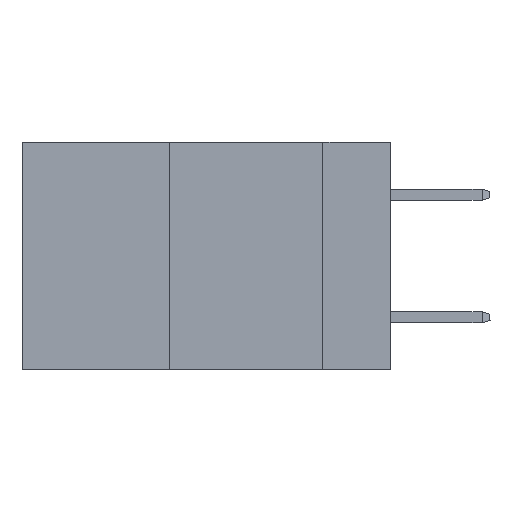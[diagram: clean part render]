
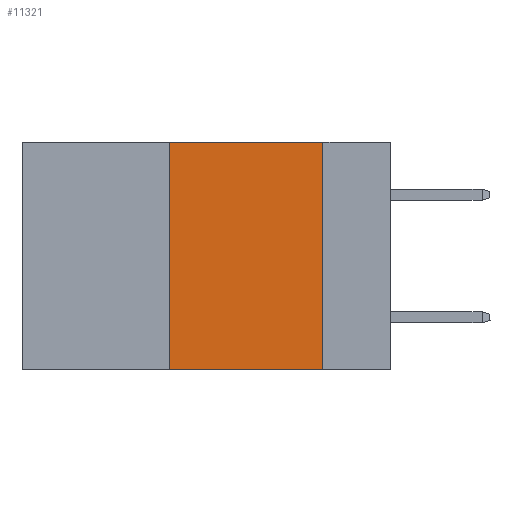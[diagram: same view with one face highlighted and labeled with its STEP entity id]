
A CAD part, left-side view. The second image highlights one B-rep face of the part: STEP entity #11321.
In plain terms, the highlighted planar face has unit normal (-1, 0, 0).
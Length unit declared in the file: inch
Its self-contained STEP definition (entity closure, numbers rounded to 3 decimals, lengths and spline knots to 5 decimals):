
#44 = LINE ( 'NONE', #5130, #1860 ) ;
#545 = CARTESIAN_POINT ( 'NONE',  ( 0., 0.6, 0. ) ) ;
#884 = EDGE_CURVE ( 'NONE', #6959, #10726, #12597, .T. ) ;
#888 = EDGE_CURVE ( 'NONE', #15827, #6959, #13977, .T. ) ;
#1541 = FACE_OUTER_BOUND ( 'NONE', #12123, .T. ) ;
#1860 = VECTOR ( 'NONE', #12966, 39.37008 ) ;
#2761 = ORIENTED_EDGE ( 'NONE', *, *, #884, .F. ) ;
#2857 = AXIS2_PLACEMENT_3D ( 'NONE', #14589, #6434, #11677 ) ;
#2940 = LINE ( 'NONE', #3061, #4414 ) ;
#3061 = CARTESIAN_POINT ( 'NONE',  ( 0., 0.6, -0.37 ) ) ;
#4271 = EDGE_CURVE ( 'NONE', #15827, #9612, #2940, .T. ) ;
#4414 = VECTOR ( 'NONE', #5964, 39.37008 ) ;
#5130 = CARTESIAN_POINT ( 'NONE',  ( 0., 0.11, 0. ) ) ;
#5546 = EDGE_CURVE ( 'NONE', #10726, #9612, #44, .T. ) ;
#5548 = ORIENTED_EDGE ( 'NONE', *, *, #888, .F. ) ;
#5964 = DIRECTION ( 'NONE',  ( 0., -1., 0. ) ) ;
#6434 = DIRECTION ( 'NONE',  ( 1., 0., 0. ) ) ;
#6959 = VERTEX_POINT ( 'NONE', #12556 ) ;
#7631 = VECTOR ( 'NONE', #11240, 39.37008 ) ;
#8489 = ORIENTED_EDGE ( 'NONE', *, *, #4271, .T. ) ;
#9612 = VERTEX_POINT ( 'NONE', #15588 ) ;
#10726 = VERTEX_POINT ( 'NONE', #15538 ) ;
#11240 = DIRECTION ( 'NONE',  ( 0., -1., 0. ) ) ;
#11321 = ADVANCED_FACE ( 'NONE', ( #1541 ), #14647, .F. ) ;
#11677 = DIRECTION ( 'NONE',  ( 0., 0., -1. ) ) ;
#12123 = EDGE_LOOP ( 'NONE', ( #16167, #2761, #5548, #8489 ) ) ;
#12556 = CARTESIAN_POINT ( 'NONE',  ( 0., 0.36, 0. ) ) ;
#12597 = LINE ( 'NONE', #545, #7631 ) ;
#12966 = DIRECTION ( 'NONE',  ( 0., 0., -1. ) ) ;
#13629 = CARTESIAN_POINT ( 'NONE',  ( 0., 0.36, -0.37 ) ) ;
#13977 = LINE ( 'NONE', #15666, #15411 ) ;
#14589 = CARTESIAN_POINT ( 'NONE',  ( 0., 0.6, 0. ) ) ;
#14647 = PLANE ( 'NONE',  #2857 ) ;
#14680 = DIRECTION ( 'NONE',  ( 0., 0., 1. ) ) ;
#15411 = VECTOR ( 'NONE', #14680, 39.37008 ) ;
#15538 = CARTESIAN_POINT ( 'NONE',  ( 0., 0.11, 0. ) ) ;
#15588 = CARTESIAN_POINT ( 'NONE',  ( 0., 0.11, -0.37 ) ) ;
#15666 = CARTESIAN_POINT ( 'NONE',  ( 0., 0.36, 0. ) ) ;
#15827 = VERTEX_POINT ( 'NONE', #13629 ) ;
#16167 = ORIENTED_EDGE ( 'NONE', *, *, #5546, .F. ) ;
